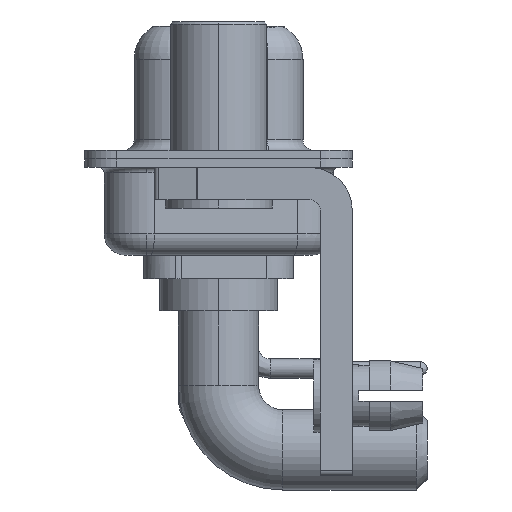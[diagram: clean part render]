
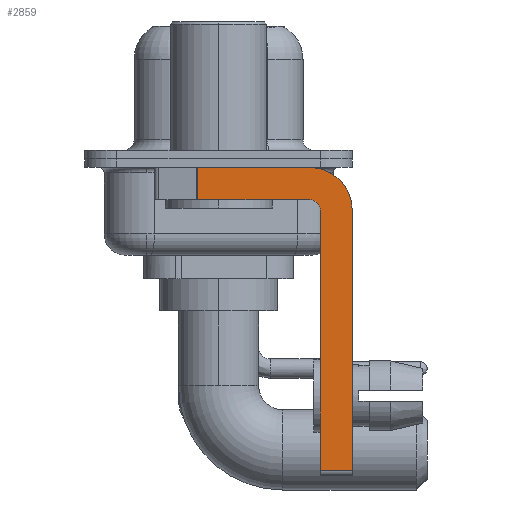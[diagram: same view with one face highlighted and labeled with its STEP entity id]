
A CAD part, left-side view. The second image highlights one B-rep face of the part: STEP entity #2859.
In plain terms, the highlighted planar face has unit normal (-1, 0, 0).
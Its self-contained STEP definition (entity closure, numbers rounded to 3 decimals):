
#38 = EDGE_CURVE ( 'NONE', #21621, #10959, #16578, .T. ) ;
#1906 = EDGE_CURVE ( 'NONE', #23828, #25346, #7559, .T. ) ;
#2445 = CARTESIAN_POINT ( 'NONE',  ( -2.9, -6.25, -2.4 ) ) ;
#2854 = VERTEX_POINT ( 'NONE', #18441 ) ;
#2859 = ADVANCED_FACE ( 'NONE', ( #9641 ), #18598, .F. ) ;
#3027 = EDGE_CURVE ( 'NONE', #26752, #23828, #11768, .T. ) ;
#3079 = VECTOR ( 'NONE', #6027, 1000. ) ;
#3437 = DIRECTION ( 'NONE',  ( 0., 0., -1. ) ) ;
#3517 = EDGE_CURVE ( 'NONE', #2854, #15085, #25709, .T. ) ;
#3946 = AXIS2_PLACEMENT_3D ( 'NONE', #28200, #12940, #8551 ) ;
#4357 = CARTESIAN_POINT ( 'NONE',  ( -2.9, 0.978, -1.9 ) ) ;
#5647 = CARTESIAN_POINT ( 'NONE',  ( -2.9, -4.75, -14.8 ) ) ;
#6027 = DIRECTION ( 'NONE',  ( 0., -1., 0. ) ) ;
#6735 = EDGE_LOOP ( 'NONE', ( #14601, #27820, #20867, #24932, #13164, #24081, #23241, #19095 ) ) ;
#7541 = CARTESIAN_POINT ( 'NONE',  ( -2.9, -4.75, -14.55 ) ) ;
#7559 = LINE ( 'NONE', #20577, #13509 ) ;
#7649 = VECTOR ( 'NONE', #12633, 1000. ) ;
#7898 = CARTESIAN_POINT ( 'NONE',  ( -2.9, -4.25, -0.4 ) ) ;
#8018 = DIRECTION ( 'NONE',  ( 1., 0., 0. ) ) ;
#8551 = DIRECTION ( 'NONE',  ( 0., 0., 1. ) ) ;
#9641 = FACE_OUTER_BOUND ( 'NONE', #6735, .T. ) ;
#10199 = EDGE_CURVE ( 'NONE', #21504, #21621, #16759, .T. ) ;
#10348 = CARTESIAN_POINT ( 'NONE',  ( -2.9, -4.25, -2.4 ) ) ;
#10744 = DIRECTION ( 'NONE',  ( 0., -1., 0. ) ) ;
#10959 = VERTEX_POINT ( 'NONE', #28473 ) ;
#11768 = CIRCLE ( 'NONE', #18795, 2. ) ;
#12633 = DIRECTION ( 'NONE',  ( 0., 0., 1. ) ) ;
#12940 = DIRECTION ( 'NONE',  ( -1., 0., 0. ) ) ;
#13164 = ORIENTED_EDGE ( 'NONE', *, *, #10199, .F. ) ;
#13509 = VECTOR ( 'NONE', #16467, 1000. ) ;
#14338 = VECTOR ( 'NONE', #26173, 1000. ) ;
#14555 = CARTESIAN_POINT ( 'NONE',  ( -2.9, 0.978, -1.9 ) ) ;
#14601 = ORIENTED_EDGE ( 'NONE', *, *, #27372, .F. ) ;
#14832 = VECTOR ( 'NONE', #10744, 1000. ) ;
#15085 = VERTEX_POINT ( 'NONE', #4357 ) ;
#15163 = LINE ( 'NONE', #17238, #14338 ) ;
#16467 = DIRECTION ( 'NONE',  ( 0., 0., -1. ) ) ;
#16578 = CIRCLE ( 'NONE', #3946, 0.5 ) ;
#16759 = LINE ( 'NONE', #5647, #7649 ) ;
#17238 = CARTESIAN_POINT ( 'NONE',  ( -2.9, -4.25, -1.9 ) ) ;
#17995 = CARTESIAN_POINT ( 'NONE',  ( -2.9, -6.25, -14.55 ) ) ;
#18116 = DIRECTION ( 'NONE',  ( 0., 0., -1. ) ) ;
#18441 = CARTESIAN_POINT ( 'NONE',  ( -2.9, 0.978, -0.4 ) ) ;
#18598 = PLANE ( 'NONE',  #25433 ) ;
#18795 = AXIS2_PLACEMENT_3D ( 'NONE', #10348, #22044, #18116 ) ;
#19095 = ORIENTED_EDGE ( 'NONE', *, *, #3027, .F. ) ;
#20577 = CARTESIAN_POINT ( 'NONE',  ( -2.9, -6.25, -2.4 ) ) ;
#20867 = ORIENTED_EDGE ( 'NONE', *, *, #26903, .F. ) ;
#20997 = CARTESIAN_POINT ( 'NONE',  ( -2.9, -4.75, -2.4 ) ) ;
#21504 = VERTEX_POINT ( 'NONE', #7541 ) ;
#21621 = VERTEX_POINT ( 'NONE', #20997 ) ;
#21710 = VECTOR ( 'NONE', #3437, 1000. ) ;
#21728 = LINE ( 'NONE', #21880, #14832 ) ;
#21839 = CARTESIAN_POINT ( 'NONE',  ( -2.9, -4.25, -14.55 ) ) ;
#21880 = CARTESIAN_POINT ( 'NONE',  ( -2.9, 3., -0.4 ) ) ;
#22044 = DIRECTION ( 'NONE',  ( 1., 0., 0. ) ) ;
#23241 = ORIENTED_EDGE ( 'NONE', *, *, #1906, .F. ) ;
#23828 = VERTEX_POINT ( 'NONE', #2445 ) ;
#24081 = ORIENTED_EDGE ( 'NONE', *, *, #24706, .T. ) ;
#24706 = EDGE_CURVE ( 'NONE', #21504, #25346, #26093, .T. ) ;
#24932 = ORIENTED_EDGE ( 'NONE', *, *, #38, .F. ) ;
#25346 = VERTEX_POINT ( 'NONE', #17995 ) ;
#25433 = AXIS2_PLACEMENT_3D ( 'NONE', #26027, #8018, #25881 ) ;
#25709 = LINE ( 'NONE', #14555, #21710 ) ;
#25881 = DIRECTION ( 'NONE',  ( 0., 0., -1. ) ) ;
#26027 = CARTESIAN_POINT ( 'NONE',  ( -2.9, -4.25, -2.4 ) ) ;
#26093 = LINE ( 'NONE', #21839, #3079 ) ;
#26173 = DIRECTION ( 'NONE',  ( 0., 1., 0. ) ) ;
#26752 = VERTEX_POINT ( 'NONE', #7898 ) ;
#26903 = EDGE_CURVE ( 'NONE', #10959, #15085, #15163, .T. ) ;
#27372 = EDGE_CURVE ( 'NONE', #2854, #26752, #21728, .T. ) ;
#27820 = ORIENTED_EDGE ( 'NONE', *, *, #3517, .T. ) ;
#28200 = CARTESIAN_POINT ( 'NONE',  ( -2.9, -4.25, -2.4 ) ) ;
#28473 = CARTESIAN_POINT ( 'NONE',  ( -2.9, -4.25, -1.9 ) ) ;
